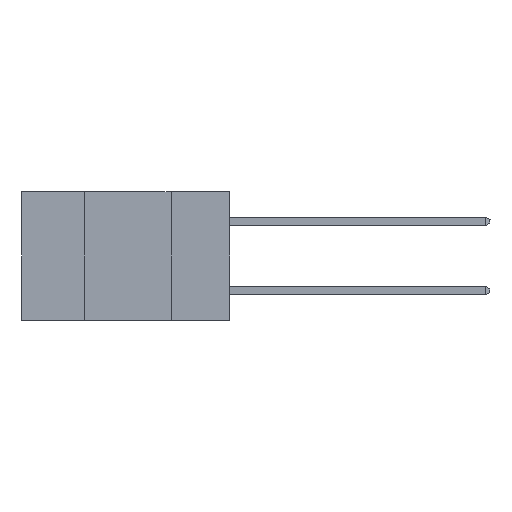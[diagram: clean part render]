
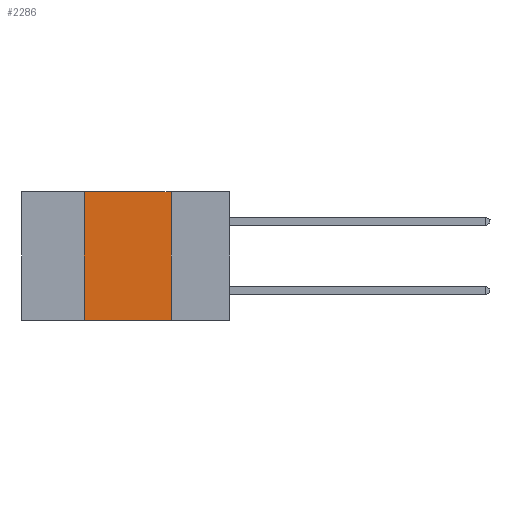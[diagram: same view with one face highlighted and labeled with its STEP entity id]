
A CAD part, left-side view. The second image highlights one B-rep face of the part: STEP entity #2286.
In plain terms, the highlighted planar face has unit normal (-1, 0, 0).
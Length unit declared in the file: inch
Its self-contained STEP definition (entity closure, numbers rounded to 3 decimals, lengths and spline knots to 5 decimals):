
#501 = ORIENTED_EDGE ( 'NONE', *, *, #10775, .T. ) ;
#1023 = LINE ( 'NONE', #14389, #11971 ) ;
#1091 = VECTOR ( 'NONE', #13149, 39.37008 ) ;
#1801 = CARTESIAN_POINT ( 'NONE',  ( 0., 0.6, 0. ) ) ;
#1822 = CARTESIAN_POINT ( 'NONE',  ( 0., 0.17, -0.37 ) ) ;
#2286 = ADVANCED_FACE ( 'NONE', ( #3828 ), #6557, .F. ) ;
#3828 = FACE_OUTER_BOUND ( 'NONE', #12851, .T. ) ;
#4334 = ORIENTED_EDGE ( 'NONE', *, *, #5334, .F. ) ;
#4521 = ORIENTED_EDGE ( 'NONE', *, *, #12002, .F. ) ;
#4877 = DIRECTION ( 'NONE',  ( 0., 0., -1. ) ) ;
#4932 = VERTEX_POINT ( 'NONE', #5245 ) ;
#5245 = CARTESIAN_POINT ( 'NONE',  ( 0., 0.42, 0. ) ) ;
#5334 = EDGE_CURVE ( 'NONE', #6737, #7448, #5400, .T. ) ;
#5400 = LINE ( 'NONE', #7546, #7164 ) ;
#6557 = PLANE ( 'NONE',  #14055 ) ;
#6737 = VERTEX_POINT ( 'NONE', #11365 ) ;
#6796 = DIRECTION ( 'NONE',  ( 0., 0., 1. ) ) ;
#6943 = DIRECTION ( 'NONE',  ( 1., 0., 0. ) ) ;
#7164 = VECTOR ( 'NONE', #4877, 39.37008 ) ;
#7177 = ORIENTED_EDGE ( 'NONE', *, *, #14356, .F. ) ;
#7448 = VERTEX_POINT ( 'NONE', #1822 ) ;
#7546 = CARTESIAN_POINT ( 'NONE',  ( 0., 0.17, 0. ) ) ;
#9708 = VECTOR ( 'NONE', #6796, 39.37008 ) ;
#10775 = EDGE_CURVE ( 'NONE', #11062, #7448, #1023, .T. ) ;
#11062 = VERTEX_POINT ( 'NONE', #11136 ) ;
#11136 = CARTESIAN_POINT ( 'NONE',  ( 0., 0.42, -0.37 ) ) ;
#11365 = CARTESIAN_POINT ( 'NONE',  ( 0., 0.17, 0. ) ) ;
#11883 = DIRECTION ( 'NONE',  ( 0., -1., 0. ) ) ;
#11971 = VECTOR ( 'NONE', #11883, 39.37008 ) ;
#12002 = EDGE_CURVE ( 'NONE', #11062, #4932, #12308, .T. ) ;
#12308 = LINE ( 'NONE', #15373, #9708 ) ;
#12851 = EDGE_LOOP ( 'NONE', ( #4334, #7177, #4521, #501 ) ) ;
#12966 = CARTESIAN_POINT ( 'NONE',  ( 0., 0.6, 0. ) ) ;
#13149 = DIRECTION ( 'NONE',  ( 0., -1., 0. ) ) ;
#13827 = DIRECTION ( 'NONE',  ( 0., 0., -1. ) ) ;
#13834 = LINE ( 'NONE', #1801, #1091 ) ;
#14055 = AXIS2_PLACEMENT_3D ( 'NONE', #12966, #6943, #13827 ) ;
#14356 = EDGE_CURVE ( 'NONE', #4932, #6737, #13834, .T. ) ;
#14389 = CARTESIAN_POINT ( 'NONE',  ( 0., 0.6, -0.37 ) ) ;
#15373 = CARTESIAN_POINT ( 'NONE',  ( 0., 0.42, 0. ) ) ;
